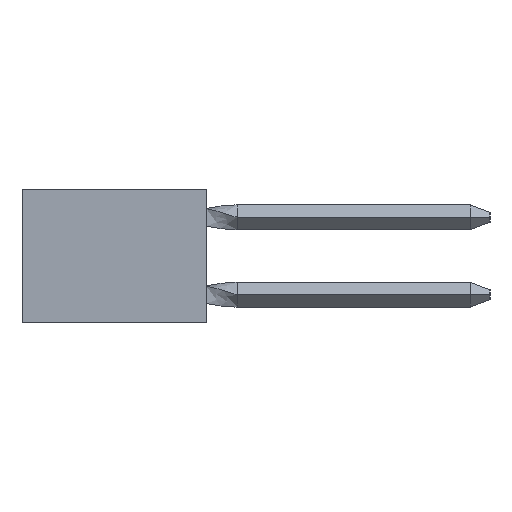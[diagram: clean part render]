
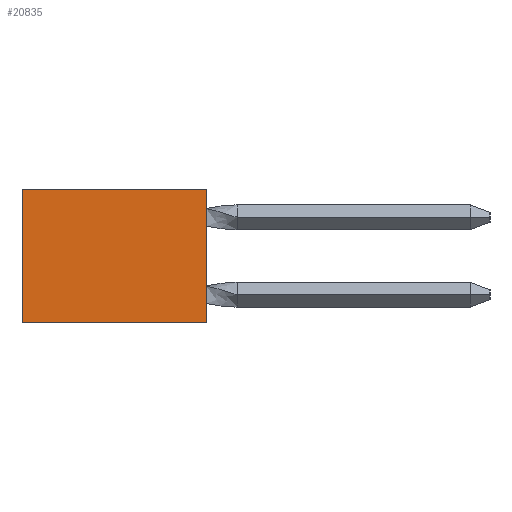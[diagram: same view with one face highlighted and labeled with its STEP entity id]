
A CAD part, left-side view. The second image highlights one B-rep face of the part: STEP entity #20835.
In plain terms, the highlighted planar face has unit normal (-1, 0, 0).
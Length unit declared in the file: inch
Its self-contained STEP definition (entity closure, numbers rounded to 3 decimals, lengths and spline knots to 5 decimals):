
#361 = DIRECTION ( 'NONE',  ( 0., 0., 1. ) ) ;
#655 = DIRECTION ( 'NONE',  ( 0., 0., -1. ) ) ;
#1590 = LINE ( 'NONE', #14892, #23697 ) ;
#1663 = VECTOR ( 'NONE', #21220, 39.37008 ) ;
#2671 = DIRECTION ( 'NONE',  ( 0., 0., -1. ) ) ;
#3460 = CARTESIAN_POINT ( 'NONE',  ( 0.298, -0.027, 0. ) ) ;
#4427 = CARTESIAN_POINT ( 'NONE',  ( 0.298, 0.473, -0.343 ) ) ;
#7395 = CARTESIAN_POINT ( 'NONE',  ( 0.298, 0., 0. ) ) ;
#7873 = VERTEX_POINT ( 'NONE', #9898 ) ;
#7874 = VERTEX_POINT ( 'NONE', #23988 ) ;
#8619 = CARTESIAN_POINT ( 'NONE',  ( 0.298, 0.473, 0. ) ) ;
#9164 = EDGE_CURVE ( 'NONE', #7873, #35306, #1590, .T. ) ;
#9898 = CARTESIAN_POINT ( 'NONE',  ( 0.298, 0., -0.343 ) ) ;
#12580 = ORIENTED_EDGE ( 'NONE', *, *, #34031, .T. ) ;
#12952 = LINE ( 'NONE', #17914, #32749 ) ;
#14892 = CARTESIAN_POINT ( 'NONE',  ( 0.298, 0., -0.343 ) ) ;
#15051 = PLANE ( 'NONE',  #16347 ) ;
#15670 = ORIENTED_EDGE ( 'NONE', *, *, #33576, .F. ) ;
#16324 = CARTESIAN_POINT ( 'NONE',  ( 0.298, 0.473, 0. ) ) ;
#16347 = AXIS2_PLACEMENT_3D ( 'NONE', #3460, #35157, #655 ) ;
#17539 = ORIENTED_EDGE ( 'NONE', *, *, #21245, .T. ) ;
#17914 = CARTESIAN_POINT ( 'NONE',  ( 0.298, -0.027, 0. ) ) ;
#19719 = LINE ( 'NONE', #4427, #1663 ) ;
#20835 = ADVANCED_FACE ( 'NONE', ( #29422 ), #15051, .F. ) ;
#21220 = DIRECTION ( 'NONE',  ( 0., 1., 0. ) ) ;
#21245 = EDGE_CURVE ( 'NONE', #33707, #7874, #37046, .T. ) ;
#22679 = VECTOR ( 'NONE', #2671, 39.37008 ) ;
#23697 = VECTOR ( 'NONE', #361, 39.37008 ) ;
#23988 = CARTESIAN_POINT ( 'NONE',  ( 0.298, 0.473, -0.343 ) ) ;
#24930 = EDGE_LOOP ( 'NONE', ( #26474, #12580, #17539, #15670 ) ) ;
#26474 = ORIENTED_EDGE ( 'NONE', *, *, #9164, .T. ) ;
#29422 = FACE_OUTER_BOUND ( 'NONE', #24930, .T. ) ;
#29607 = DIRECTION ( 'NONE',  ( 0., 1., 0. ) ) ;
#32749 = VECTOR ( 'NONE', #29607, 39.37008 ) ;
#33576 = EDGE_CURVE ( 'NONE', #7873, #7874, #19719, .T. ) ;
#33707 = VERTEX_POINT ( 'NONE', #16324 ) ;
#34031 = EDGE_CURVE ( 'NONE', #35306, #33707, #12952, .T. ) ;
#35157 = DIRECTION ( 'NONE',  ( 1., 0., 0. ) ) ;
#35306 = VERTEX_POINT ( 'NONE', #7395 ) ;
#37046 = LINE ( 'NONE', #8619, #22679 ) ;
